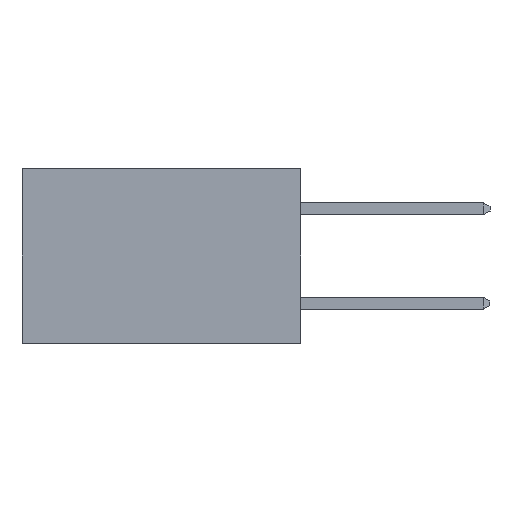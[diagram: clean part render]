
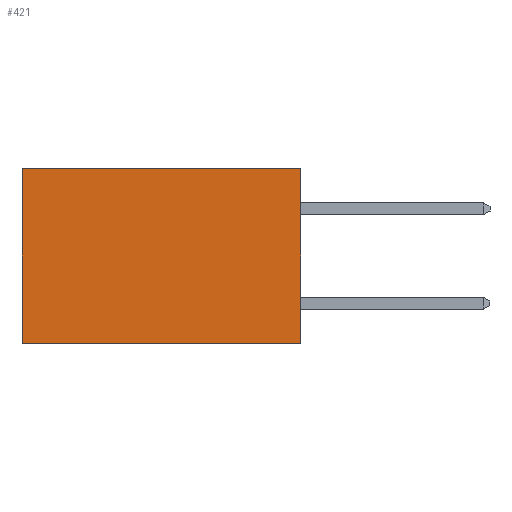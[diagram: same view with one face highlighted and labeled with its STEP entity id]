
A CAD part, left-side view. The second image highlights one B-rep face of the part: STEP entity #421.
In plain terms, the highlighted planar face has unit normal (-1, 0, 0).
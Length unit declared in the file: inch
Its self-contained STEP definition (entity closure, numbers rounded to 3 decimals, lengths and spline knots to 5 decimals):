
#214 = LINE ( 'NONE', #1482, #8723 ) ;
#280 = ORIENTED_EDGE ( 'NONE', *, *, #8548, .F. ) ;
#421 = ADVANCED_FACE ( 'NONE', ( #2956 ), #9830, .F. ) ;
#1119 = AXIS2_PLACEMENT_3D ( 'NONE', #8378, #1421, #7871 ) ;
#1421 = DIRECTION ( 'NONE',  ( 1., 0., 0. ) ) ;
#1482 = CARTESIAN_POINT ( 'NONE',  ( 0.277, 0., -0.37 ) ) ;
#1540 = VECTOR ( 'NONE', #4280, 39.37008 ) ;
#1977 = CARTESIAN_POINT ( 'NONE',  ( 0.277, 0., -0.37 ) ) ;
#2505 = ORIENTED_EDGE ( 'NONE', *, *, #3563, .T. ) ;
#2775 = ORIENTED_EDGE ( 'NONE', *, *, #10995, .T. ) ;
#2891 = CARTESIAN_POINT ( 'NONE',  ( 0.277, 0.59, -0.37 ) ) ;
#2956 = FACE_OUTER_BOUND ( 'NONE', #4140, .T. ) ;
#3026 = VERTEX_POINT ( 'NONE', #7375 ) ;
#3420 = CARTESIAN_POINT ( 'NONE',  ( 0.277, 0., 0. ) ) ;
#3563 = EDGE_CURVE ( 'NONE', #9751, #5595, #8681, .T. ) ;
#4140 = EDGE_LOOP ( 'NONE', ( #2505, #4809, #280, #2775 ) ) ;
#4280 = DIRECTION ( 'NONE',  ( 0., 1., 0. ) ) ;
#4809 = ORIENTED_EDGE ( 'NONE', *, *, #8060, .F. ) ;
#5343 = DIRECTION ( 'NONE',  ( 0., 0., -1. ) ) ;
#5595 = VERTEX_POINT ( 'NONE', #2891 ) ;
#6383 = VECTOR ( 'NONE', #5343, 39.37008 ) ;
#6431 = LINE ( 'NONE', #1977, #10690 ) ;
#6559 = CARTESIAN_POINT ( 'NONE',  ( 0.277, 0.59, -0.37 ) ) ;
#7375 = CARTESIAN_POINT ( 'NONE',  ( 0.277, 0., -0.37 ) ) ;
#7720 = VERTEX_POINT ( 'NONE', #10962 ) ;
#7871 = DIRECTION ( 'NONE',  ( 0., 0., -1. ) ) ;
#7952 = DIRECTION ( 'NONE',  ( 0., 1., 0. ) ) ;
#8060 = EDGE_CURVE ( 'NONE', #3026, #5595, #6431, .T. ) ;
#8378 = CARTESIAN_POINT ( 'NONE',  ( 0.277, 0., -0.37 ) ) ;
#8420 = LINE ( 'NONE', #3420, #1540 ) ;
#8548 = EDGE_CURVE ( 'NONE', #7720, #3026, #214, .T. ) ;
#8681 = LINE ( 'NONE', #6559, #6383 ) ;
#8723 = VECTOR ( 'NONE', #9263, 39.37008 ) ;
#9263 = DIRECTION ( 'NONE',  ( 0., 0., -1. ) ) ;
#9751 = VERTEX_POINT ( 'NONE', #11220 ) ;
#9830 = PLANE ( 'NONE',  #1119 ) ;
#10690 = VECTOR ( 'NONE', #7952, 39.37008 ) ;
#10962 = CARTESIAN_POINT ( 'NONE',  ( 0.277, 0., 0. ) ) ;
#10995 = EDGE_CURVE ( 'NONE', #7720, #9751, #8420, .T. ) ;
#11220 = CARTESIAN_POINT ( 'NONE',  ( 0.277, 0.59, 0. ) ) ;
